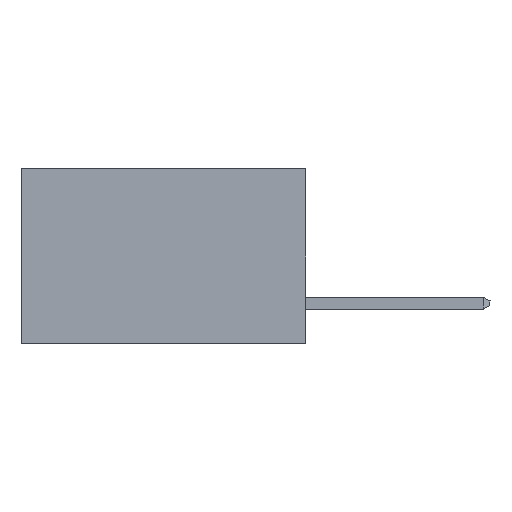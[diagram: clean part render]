
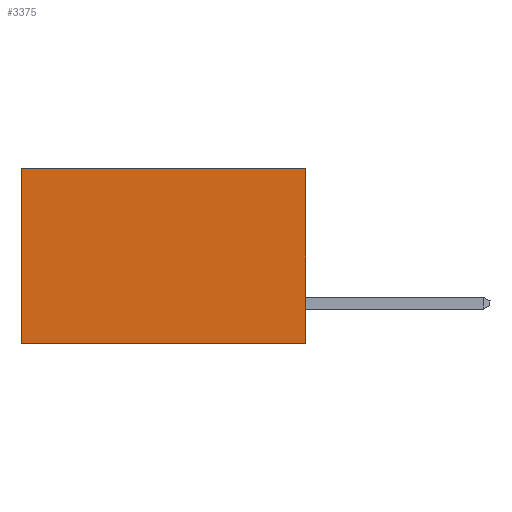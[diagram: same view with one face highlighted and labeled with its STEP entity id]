
A CAD part, left-side view. The second image highlights one B-rep face of the part: STEP entity #3375.
In plain terms, the highlighted planar face has unit normal (-1, 0, 0).
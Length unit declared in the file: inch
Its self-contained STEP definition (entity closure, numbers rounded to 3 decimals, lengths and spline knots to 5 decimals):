
#632 = CARTESIAN_POINT ( 'NONE',  ( 0.2615, 0., 0. ) ) ;
#1925 = CARTESIAN_POINT ( 'NONE',  ( 0.2615, 0., 0. ) ) ;
#2365 = EDGE_CURVE ( 'NONE', #14202, #12735, #7666, .T. ) ;
#2423 = DIRECTION ( 'NONE',  ( 0., 0., -1. ) ) ;
#2566 = CARTESIAN_POINT ( 'NONE',  ( 0.2615, 0., -0.37 ) ) ;
#2969 = EDGE_CURVE ( 'NONE', #14202, #3875, #11081, .T. ) ;
#3375 = ADVANCED_FACE ( 'NONE', ( #16720 ), #6483, .F. ) ;
#3686 = CARTESIAN_POINT ( 'NONE',  ( 0.2615, 0., -0.37 ) ) ;
#3832 = VECTOR ( 'NONE', #9450, 39.37008 ) ;
#3842 = VECTOR ( 'NONE', #2423, 39.37008 ) ;
#3875 = VERTEX_POINT ( 'NONE', #2566 ) ;
#5164 = DIRECTION ( 'NONE',  ( 1., 0., 0. ) ) ;
#6483 = PLANE ( 'NONE',  #7279 ) ;
#6524 = EDGE_CURVE ( 'NONE', #12735, #16772, #15389, .T. ) ;
#6570 = LINE ( 'NONE', #16906, #3832 ) ;
#7279 = AXIS2_PLACEMENT_3D ( 'NONE', #9254, #5164, #16444 ) ;
#7350 = ORIENTED_EDGE ( 'NONE', *, *, #6524, .T. ) ;
#7666 = LINE ( 'NONE', #1925, #9991 ) ;
#8628 = ORIENTED_EDGE ( 'NONE', *, *, #12720, .F. ) ;
#8848 = CARTESIAN_POINT ( 'NONE',  ( 0.2615, 0.6, 0. ) ) ;
#9254 = CARTESIAN_POINT ( 'NONE',  ( 0.2615, 0., -0.37 ) ) ;
#9450 = DIRECTION ( 'NONE',  ( 0., 1., 0. ) ) ;
#9661 = DIRECTION ( 'NONE',  ( 0., 0., -1. ) ) ;
#9991 = VECTOR ( 'NONE', #17988, 39.37008 ) ;
#10665 = EDGE_LOOP ( 'NONE', ( #7350, #8628, #14528, #14447 ) ) ;
#11081 = LINE ( 'NONE', #3686, #15568 ) ;
#12720 = EDGE_CURVE ( 'NONE', #3875, #16772, #6570, .T. ) ;
#12735 = VERTEX_POINT ( 'NONE', #8848 ) ;
#14202 = VERTEX_POINT ( 'NONE', #632 ) ;
#14447 = ORIENTED_EDGE ( 'NONE', *, *, #2365, .T. ) ;
#14528 = ORIENTED_EDGE ( 'NONE', *, *, #2969, .F. ) ;
#15389 = LINE ( 'NONE', #17938, #3842 ) ;
#15568 = VECTOR ( 'NONE', #9661, 39.37008 ) ;
#16444 = DIRECTION ( 'NONE',  ( 0., 0., -1. ) ) ;
#16720 = FACE_OUTER_BOUND ( 'NONE', #10665, .T. ) ;
#16772 = VERTEX_POINT ( 'NONE', #18680 ) ;
#16906 = CARTESIAN_POINT ( 'NONE',  ( 0.2615, 0., -0.37 ) ) ;
#17938 = CARTESIAN_POINT ( 'NONE',  ( 0.2615, 0.6, -0.37 ) ) ;
#17988 = DIRECTION ( 'NONE',  ( 0., 1., 0. ) ) ;
#18680 = CARTESIAN_POINT ( 'NONE',  ( 0.2615, 0.6, -0.37 ) ) ;
